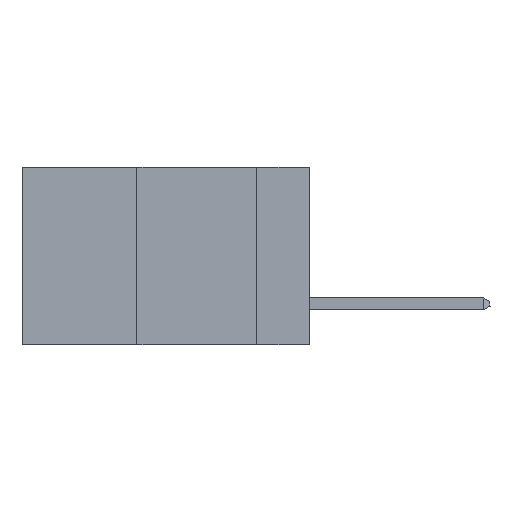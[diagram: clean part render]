
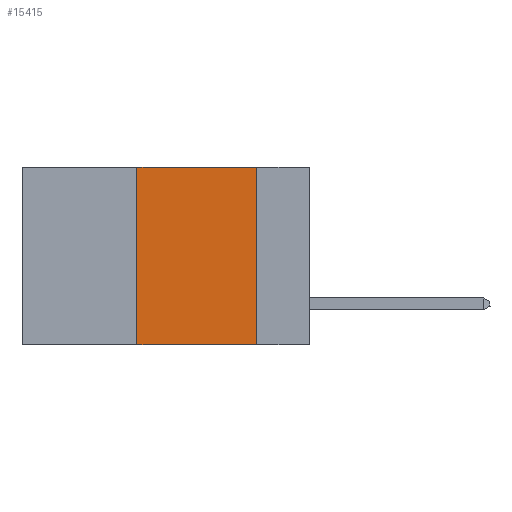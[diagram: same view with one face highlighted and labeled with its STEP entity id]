
A CAD part, left-side view. The second image highlights one B-rep face of the part: STEP entity #15415.
In plain terms, the highlighted planar face has unit normal (-1, 0, 0).
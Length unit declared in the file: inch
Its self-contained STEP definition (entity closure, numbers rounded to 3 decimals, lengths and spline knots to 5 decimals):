
#495 = CARTESIAN_POINT ( 'NONE',  ( 0., 0.11, 0. ) ) ;
#1078 = CARTESIAN_POINT ( 'NONE',  ( 0., 0.11, -0.37 ) ) ;
#2172 = CARTESIAN_POINT ( 'NONE',  ( 0., 0.36, 0. ) ) ;
#3098 = DIRECTION ( 'NONE',  ( 1., 0., 0. ) ) ;
#3385 = LINE ( 'NONE', #29126, #31946 ) ;
#4398 = EDGE_CURVE ( 'NONE', #21098, #4431, #27022, .T. ) ;
#4431 = VERTEX_POINT ( 'NONE', #1078 ) ;
#4649 = ORIENTED_EDGE ( 'NONE', *, *, #20061, .F. ) ;
#9155 = CARTESIAN_POINT ( 'NONE',  ( 0., 0.36, 0. ) ) ;
#10051 = FACE_OUTER_BOUND ( 'NONE', #17752, .T. ) ;
#10214 = VECTOR ( 'NONE', #20506, 39.37008 ) ;
#10871 = CARTESIAN_POINT ( 'NONE',  ( 0., 0.36, -0.37 ) ) ;
#14142 = ORIENTED_EDGE ( 'NONE', *, *, #28680, .F. ) ;
#15415 = ADVANCED_FACE ( 'NONE', ( #10051 ), #28402, .F. ) ;
#17281 = LINE ( 'NONE', #9155, #22347 ) ;
#17752 = EDGE_LOOP ( 'NONE', ( #30155, #4649, #14142, #27837 ) ) ;
#19563 = VECTOR ( 'NONE', #31228, 39.37008 ) ;
#19876 = VERTEX_POINT ( 'NONE', #2172 ) ;
#20061 = EDGE_CURVE ( 'NONE', #19876, #26801, #3385, .T. ) ;
#20506 = DIRECTION ( 'NONE',  ( 0., 0., -1. ) ) ;
#20970 = CARTESIAN_POINT ( 'NONE',  ( 0., 0.6, -0.37 ) ) ;
#21098 = VERTEX_POINT ( 'NONE', #10871 ) ;
#21361 = DIRECTION ( 'NONE',  ( 0., 0., -1. ) ) ;
#22347 = VECTOR ( 'NONE', #29175, 39.37008 ) ;
#26789 = DIRECTION ( 'NONE',  ( 0., -1., 0. ) ) ;
#26801 = VERTEX_POINT ( 'NONE', #27979 ) ;
#27022 = LINE ( 'NONE', #20970, #19563 ) ;
#27837 = ORIENTED_EDGE ( 'NONE', *, *, #4398, .T. ) ;
#27979 = CARTESIAN_POINT ( 'NONE',  ( 0., 0.11, 0. ) ) ;
#28402 = PLANE ( 'NONE',  #31667 ) ;
#28517 = CARTESIAN_POINT ( 'NONE',  ( 0., 0.6, 0. ) ) ;
#28680 = EDGE_CURVE ( 'NONE', #21098, #19876, #17281, .T. ) ;
#29126 = CARTESIAN_POINT ( 'NONE',  ( 0., 0.6, 0. ) ) ;
#29175 = DIRECTION ( 'NONE',  ( 0., 0., 1. ) ) ;
#30155 = ORIENTED_EDGE ( 'NONE', *, *, #31338, .F. ) ;
#31228 = DIRECTION ( 'NONE',  ( 0., -1., 0. ) ) ;
#31338 = EDGE_CURVE ( 'NONE', #26801, #4431, #31402, .T. ) ;
#31402 = LINE ( 'NONE', #495, #10214 ) ;
#31667 = AXIS2_PLACEMENT_3D ( 'NONE', #28517, #3098, #21361 ) ;
#31946 = VECTOR ( 'NONE', #26789, 39.37008 ) ;
